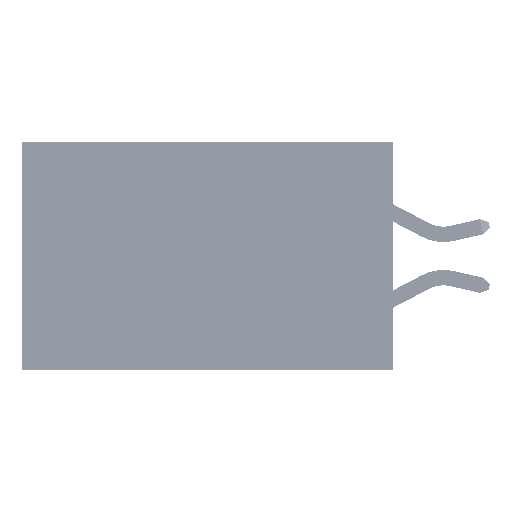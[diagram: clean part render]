
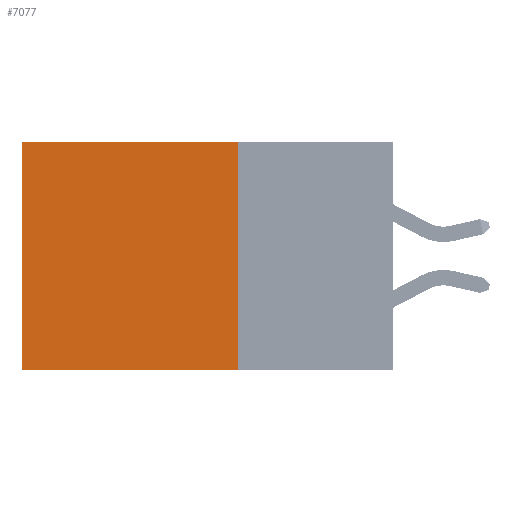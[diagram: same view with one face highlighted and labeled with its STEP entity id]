
A CAD part, left-side view. The second image highlights one B-rep face of the part: STEP entity #7077.
In plain terms, the highlighted planar face has unit normal (-1, 0, 0).
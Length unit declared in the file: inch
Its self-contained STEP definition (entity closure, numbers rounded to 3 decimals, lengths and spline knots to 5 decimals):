
#2364 = VERTEX_POINT ( 'NONE', #27980 ) ;
#3485 = CARTESIAN_POINT ( 'NONE',  ( 0.2875, 0.25, -0.37 ) ) ;
#4575 = CARTESIAN_POINT ( 'NONE',  ( 0.2875, 0.25, 0. ) ) ;
#4680 = EDGE_CURVE ( 'NONE', #35269, #2364, #28437, .T. ) ;
#6024 = EDGE_LOOP ( 'NONE', ( #23627, #41792, #12725, #9818 ) ) ;
#7077 = ADVANCED_FACE ( 'NONE', ( #19434 ), #23931, .F. ) ;
#7204 = DIRECTION ( 'NONE',  ( 0., 1., 0. ) ) ;
#9818 = ORIENTED_EDGE ( 'NONE', *, *, #13133, .T. ) ;
#9828 = DIRECTION ( 'NONE',  ( 1., 0., 0. ) ) ;
#10087 = CARTESIAN_POINT ( 'NONE',  ( 0.2875, 0.6, 0. ) ) ;
#10295 = CARTESIAN_POINT ( 'NONE',  ( 0.2875, 0.25, 0. ) ) ;
#12725 = ORIENTED_EDGE ( 'NONE', *, *, #13911, .F. ) ;
#13133 = EDGE_CURVE ( 'NONE', #17861, #19498, #42215, .T. ) ;
#13911 = EDGE_CURVE ( 'NONE', #17861, #35269, #46097, .T. ) ;
#14242 = VECTOR ( 'NONE', #18059, 39.37008 ) ;
#14475 = CARTESIAN_POINT ( 'NONE',  ( 0.2875, 0.25, 0. ) ) ;
#17179 = DIRECTION ( 'NONE',  ( 0., 1., 0. ) ) ;
#17861 = VERTEX_POINT ( 'NONE', #4575 ) ;
#18059 = DIRECTION ( 'NONE',  ( 0., 0., -1. ) ) ;
#18249 = VECTOR ( 'NONE', #42056, 39.37008 ) ;
#19434 = FACE_OUTER_BOUND ( 'NONE', #6024, .T. ) ;
#19498 = VERTEX_POINT ( 'NONE', #31942 ) ;
#21547 = AXIS2_PLACEMENT_3D ( 'NONE', #10295, #9828, #27692 ) ;
#22643 = VECTOR ( 'NONE', #17179, 39.37008 ) ;
#23627 = ORIENTED_EDGE ( 'NONE', *, *, #39618, .T. ) ;
#23931 = PLANE ( 'NONE',  #21547 ) ;
#27692 = DIRECTION ( 'NONE',  ( 0., 0., -1. ) ) ;
#27872 = VECTOR ( 'NONE', #7204, 39.37008 ) ;
#27980 = CARTESIAN_POINT ( 'NONE',  ( 0.2875, 0.6, -0.37 ) ) ;
#28437 = LINE ( 'NONE', #3485, #27872 ) ;
#31942 = CARTESIAN_POINT ( 'NONE',  ( 0.2875, 0.6, 0. ) ) ;
#35269 = VERTEX_POINT ( 'NONE', #37285 ) ;
#37238 = LINE ( 'NONE', #10087, #18249 ) ;
#37285 = CARTESIAN_POINT ( 'NONE',  ( 0.2875, 0.25, -0.37 ) ) ;
#38559 = CARTESIAN_POINT ( 'NONE',  ( 0.2875, 0.25, 0. ) ) ;
#39618 = EDGE_CURVE ( 'NONE', #19498, #2364, #37238, .T. ) ;
#41792 = ORIENTED_EDGE ( 'NONE', *, *, #4680, .F. ) ;
#42056 = DIRECTION ( 'NONE',  ( 0., 0., -1. ) ) ;
#42215 = LINE ( 'NONE', #38559, #22643 ) ;
#46097 = LINE ( 'NONE', #14475, #14242 ) ;
